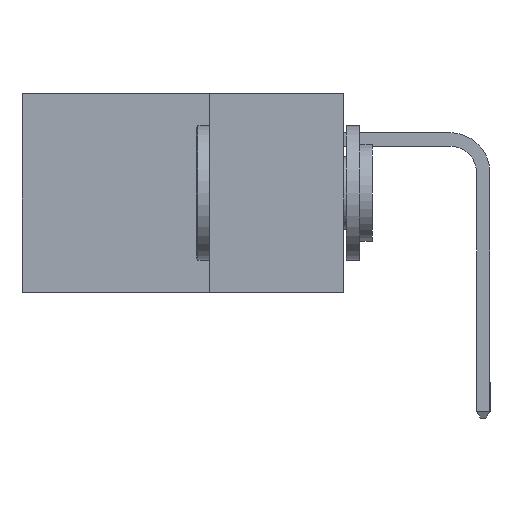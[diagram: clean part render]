
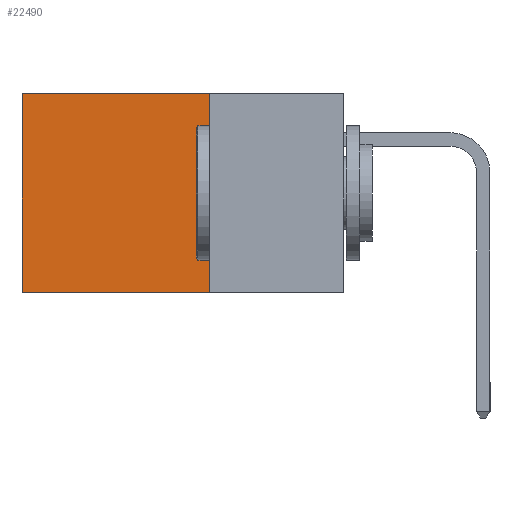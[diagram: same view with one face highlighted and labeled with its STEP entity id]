
A CAD part, left-side view. The second image highlights one B-rep face of the part: STEP entity #22490.
In plain terms, the highlighted planar face has unit normal (-1, 0, 0).
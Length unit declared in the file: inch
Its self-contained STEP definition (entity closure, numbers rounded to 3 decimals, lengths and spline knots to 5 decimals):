
#2282 = EDGE_LOOP ( 'NONE', ( #20218, #4791, #25952, #3723 ) ) ;
#3723 = ORIENTED_EDGE ( 'NONE', *, *, #26141, .T. ) ;
#3758 = EDGE_CURVE ( 'NONE', #27321, #16992, #20939, .T. ) ;
#4113 = DIRECTION ( 'NONE',  ( 0., 0., -1. ) ) ;
#4791 = ORIENTED_EDGE ( 'NONE', *, *, #25376, .F. ) ;
#7891 = DIRECTION ( 'NONE',  ( 0., 0., -1. ) ) ;
#8140 = CARTESIAN_POINT ( 'NONE',  ( 0.298, 0.6, 0. ) ) ;
#9760 = DIRECTION ( 'NONE',  ( 0., 1., 0. ) ) ;
#11967 = VECTOR ( 'NONE', #19282, 39.37008 ) ;
#12123 = PLANE ( 'NONE',  #26098 ) ;
#12955 = CARTESIAN_POINT ( 'NONE',  ( 0.298, 0.25, 0. ) ) ;
#14155 = CARTESIAN_POINT ( 'NONE',  ( 0.298, 0.25, 0. ) ) ;
#14314 = FACE_OUTER_BOUND ( 'NONE', #2282, .T. ) ;
#14834 = CARTESIAN_POINT ( 'NONE',  ( 0.298, 0.25, -0.37 ) ) ;
#15928 = VECTOR ( 'NONE', #9760, 39.37008 ) ;
#16925 = VECTOR ( 'NONE', #4113, 39.37008 ) ;
#16992 = VERTEX_POINT ( 'NONE', #22275 ) ;
#17505 = CARTESIAN_POINT ( 'NONE',  ( 0.298, 0.25, -0.37 ) ) ;
#18433 = CARTESIAN_POINT ( 'NONE',  ( 0.298, 0.25, 0. ) ) ;
#18500 = EDGE_CURVE ( 'NONE', #22731, #26897, #20834, .T. ) ;
#19282 = DIRECTION ( 'NONE',  ( 0., 1., 0. ) ) ;
#19696 = CARTESIAN_POINT ( 'NONE',  ( 0.298, 0.6, 0. ) ) ;
#20218 = ORIENTED_EDGE ( 'NONE', *, *, #3758, .T. ) ;
#20604 = LINE ( 'NONE', #14834, #11967 ) ;
#20834 = LINE ( 'NONE', #14155, #21500 ) ;
#20939 = LINE ( 'NONE', #8140, #16925 ) ;
#21500 = VECTOR ( 'NONE', #22815, 39.37008 ) ;
#22242 = LINE ( 'NONE', #26557, #15928 ) ;
#22275 = CARTESIAN_POINT ( 'NONE',  ( 0.298, 0.6, -0.37 ) ) ;
#22490 = ADVANCED_FACE ( 'NONE', ( #14314 ), #12123, .F. ) ;
#22731 = VERTEX_POINT ( 'NONE', #12955 ) ;
#22815 = DIRECTION ( 'NONE',  ( 0., 0., -1. ) ) ;
#22826 = DIRECTION ( 'NONE',  ( 1., 0., 0. ) ) ;
#25376 = EDGE_CURVE ( 'NONE', #26897, #16992, #20604, .T. ) ;
#25952 = ORIENTED_EDGE ( 'NONE', *, *, #18500, .F. ) ;
#26098 = AXIS2_PLACEMENT_3D ( 'NONE', #18433, #22826, #7891 ) ;
#26141 = EDGE_CURVE ( 'NONE', #22731, #27321, #22242, .T. ) ;
#26557 = CARTESIAN_POINT ( 'NONE',  ( 0.298, 0.25, 0. ) ) ;
#26897 = VERTEX_POINT ( 'NONE', #17505 ) ;
#27321 = VERTEX_POINT ( 'NONE', #19696 ) ;
